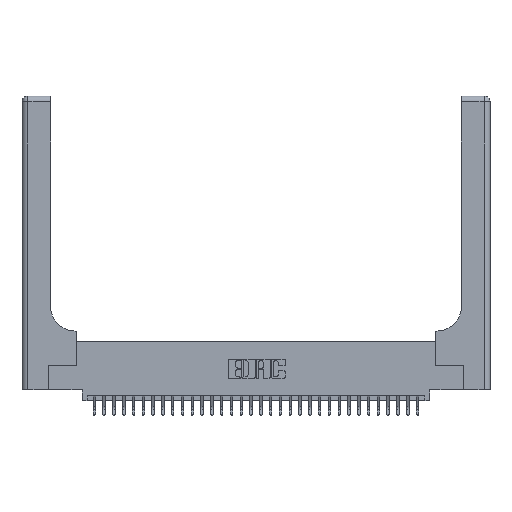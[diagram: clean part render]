
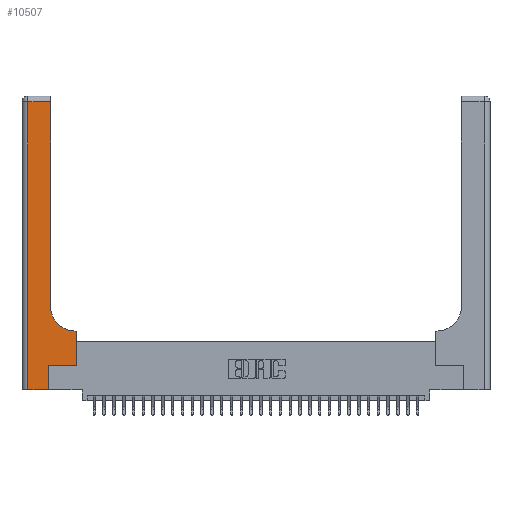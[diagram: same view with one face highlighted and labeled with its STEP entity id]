
A CAD part, top view. The second image highlights one B-rep face of the part: STEP entity #10507.
In plain terms, the highlighted planar face has unit normal (0, 0, 1).
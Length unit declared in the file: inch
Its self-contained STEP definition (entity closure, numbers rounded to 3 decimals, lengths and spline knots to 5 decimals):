
#110 = EDGE_CURVE ( 'NONE', #10584, #3594, #22646, .T. ) ;
#365 = DIRECTION ( 'NONE',  ( 1., 0., 0. ) ) ;
#932 = DIRECTION ( 'NONE',  ( 0., -1., 0. ) ) ;
#2030 = EDGE_CURVE ( 'NONE', #31518, #19040, #20927, .T. ) ;
#2104 = VECTOR ( 'NONE', #19066, 39.37008 ) ;
#2443 = CARTESIAN_POINT ( 'NONE',  ( 0.2915, 0.85, 0.37 ) ) ;
#2923 = CARTESIAN_POINT ( 'NONE',  ( 0.2915, 3., 0.37 ) ) ;
#3461 = CARTESIAN_POINT ( 'NONE',  ( 0., 2.94, 0.37 ) ) ;
#3516 = CARTESIAN_POINT ( 'NONE',  ( 0.5585, 0.6, 0.37 ) ) ;
#3594 = VERTEX_POINT ( 'NONE', #11600 ) ;
#3703 = ORIENTED_EDGE ( 'NONE', *, *, #16710, .T. ) ;
#4293 = EDGE_CURVE ( 'NONE', #26756, #30050, #6876, .T. ) ;
#4852 = DIRECTION ( 'NONE',  ( 0., 0., -1. ) ) ;
#5431 = ORIENTED_EDGE ( 'NONE', *, *, #4293, .T. ) ;
#5557 = CARTESIAN_POINT ( 'NONE',  ( 0.269, 0.25, 0.37 ) ) ;
#5562 = VECTOR ( 'NONE', #932, 39.37008 ) ;
#5754 = EDGE_CURVE ( 'NONE', #7145, #10584, #26502, .T. ) ;
#5995 = LINE ( 'NONE', #3461, #25733 ) ;
#6039 = EDGE_CURVE ( 'NONE', #30050, #29640, #10791, .T. ) ;
#6062 = DIRECTION ( 'NONE',  ( -1., 0., 0. ) ) ;
#6390 = ORIENTED_EDGE ( 'NONE', *, *, #9337, .T. ) ;
#6804 = EDGE_LOOP ( 'NONE', ( #21086, #26553, #3703, #28790, #21834, #6390, #21200, #13255, #5431 ) ) ;
#6876 = CIRCLE ( 'NONE', #27262, 0.25 ) ;
#7145 = VERTEX_POINT ( 'NONE', #30063 ) ;
#8731 = CARTESIAN_POINT ( 'NONE',  ( 0., 3., 0.37 ) ) ;
#9232 = VECTOR ( 'NONE', #21032, 39.37008 ) ;
#9337 = EDGE_CURVE ( 'NONE', #3594, #31518, #11905, .T. ) ;
#9974 = AXIS2_PLACEMENT_3D ( 'NONE', #8731, #26702, #11295 ) ;
#10507 = ADVANCED_FACE ( 'NONE', ( #13071 ), #21541, .F. ) ;
#10584 = VERTEX_POINT ( 'NONE', #11984 ) ;
#10791 = LINE ( 'NONE', #2923, #16809 ) ;
#11295 = DIRECTION ( 'NONE',  ( -1., 0., 0. ) ) ;
#11600 = CARTESIAN_POINT ( 'NONE',  ( 0.269, 0.25, 0.37 ) ) ;
#11905 = LINE ( 'NONE', #5557, #31625 ) ;
#11984 = CARTESIAN_POINT ( 'NONE',  ( 0.269, 0., 0.37 ) ) ;
#13071 = FACE_OUTER_BOUND ( 'NONE', #6804, .T. ) ;
#13255 = ORIENTED_EDGE ( 'NONE', *, *, #15910, .T. ) ;
#14244 = CARTESIAN_POINT ( 'NONE',  ( 0.5415, 0.6, 0.37 ) ) ;
#15773 = CARTESIAN_POINT ( 'NONE',  ( 0.5585, 0.25, 0.37 ) ) ;
#15910 = EDGE_CURVE ( 'NONE', #19040, #26756, #17689, .T. ) ;
#16041 = EDGE_CURVE ( 'NONE', #29640, #29010, #5995, .T. ) ;
#16710 = EDGE_CURVE ( 'NONE', #29010, #7145, #19233, .T. ) ;
#16809 = VECTOR ( 'NONE', #26123, 39.37008 ) ;
#17689 = LINE ( 'NONE', #26108, #9232 ) ;
#17953 = CARTESIAN_POINT ( 'NONE',  ( 0.06, 2.94, 0.37 ) ) ;
#18233 = DIRECTION ( 'NONE',  ( 0., 1., 0. ) ) ;
#19040 = VERTEX_POINT ( 'NONE', #3516 ) ;
#19066 = DIRECTION ( 'NONE',  ( 0., 1., 0. ) ) ;
#19233 = LINE ( 'NONE', #31763, #5562 ) ;
#19656 = VECTOR ( 'NONE', #22405, 39.37008 ) ;
#20259 = CARTESIAN_POINT ( 'NONE',  ( 0.5415, 0.85, 0.37 ) ) ;
#20927 = LINE ( 'NONE', #28468, #26941 ) ;
#21032 = DIRECTION ( 'NONE',  ( -1., 0., 0. ) ) ;
#21086 = ORIENTED_EDGE ( 'NONE', *, *, #6039, .T. ) ;
#21200 = ORIENTED_EDGE ( 'NONE', *, *, #2030, .T. ) ;
#21541 = PLANE ( 'NONE',  #9974 ) ;
#21650 = CARTESIAN_POINT ( 'NONE',  ( 0.269, 0., 0.37 ) ) ;
#21834 = ORIENTED_EDGE ( 'NONE', *, *, #110, .T. ) ;
#22405 = DIRECTION ( 'NONE',  ( 1., 0., 0. ) ) ;
#22646 = LINE ( 'NONE', #21650, #2104 ) ;
#22854 = DIRECTION ( 'NONE',  ( 1., 0., 0. ) ) ;
#25733 = VECTOR ( 'NONE', #6062, 39.37008 ) ;
#26108 = CARTESIAN_POINT ( 'NONE',  ( 0.2915, 0.6, 0.37 ) ) ;
#26123 = DIRECTION ( 'NONE',  ( 0., 1., 0. ) ) ;
#26502 = LINE ( 'NONE', #30054, #19656 ) ;
#26553 = ORIENTED_EDGE ( 'NONE', *, *, #16041, .T. ) ;
#26702 = DIRECTION ( 'NONE',  ( 0., 0., -1. ) ) ;
#26756 = VERTEX_POINT ( 'NONE', #14244 ) ;
#26941 = VECTOR ( 'NONE', #18233, 39.37008 ) ;
#27262 = AXIS2_PLACEMENT_3D ( 'NONE', #20259, #4852, #22854 ) ;
#28468 = CARTESIAN_POINT ( 'NONE',  ( 0.5585, 0.25, 0.37 ) ) ;
#28790 = ORIENTED_EDGE ( 'NONE', *, *, #5754, .T. ) ;
#29010 = VERTEX_POINT ( 'NONE', #17953 ) ;
#29640 = VERTEX_POINT ( 'NONE', #30603 ) ;
#30050 = VERTEX_POINT ( 'NONE', #2443 ) ;
#30054 = CARTESIAN_POINT ( 'NONE',  ( 0., 0., 0.37 ) ) ;
#30063 = CARTESIAN_POINT ( 'NONE',  ( 0.06, 0., 0.37 ) ) ;
#30603 = CARTESIAN_POINT ( 'NONE',  ( 0.2915, 2.94, 0.37 ) ) ;
#31518 = VERTEX_POINT ( 'NONE', #15773 ) ;
#31625 = VECTOR ( 'NONE', #365, 39.37008 ) ;
#31763 = CARTESIAN_POINT ( 'NONE',  ( 0.06, 3., 0.37 ) ) ;
